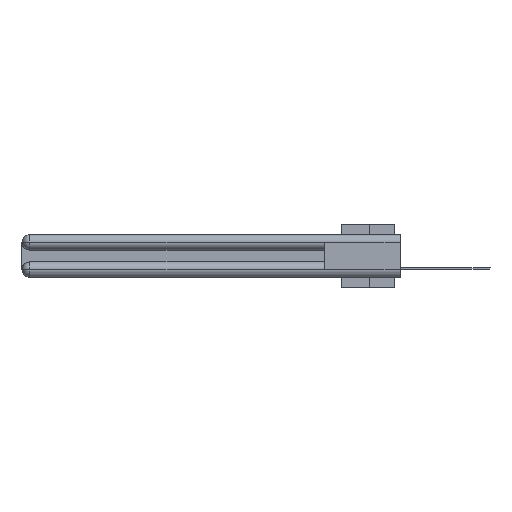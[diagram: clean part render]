
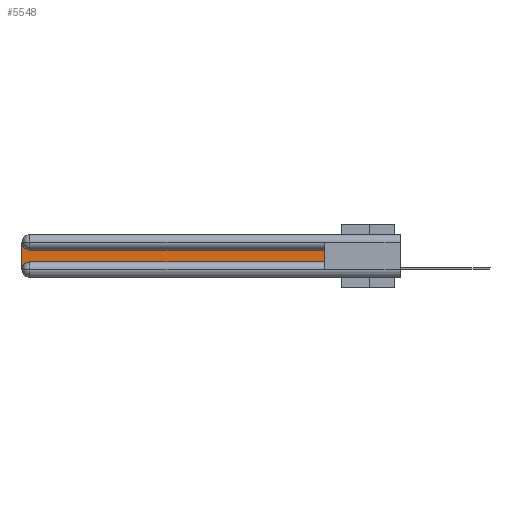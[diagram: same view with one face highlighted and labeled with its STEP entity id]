
A CAD part, left-side view. The second image highlights one B-rep face of the part: STEP entity #5548.
In plain terms, the highlighted planar face has unit normal (-1, 0, 0).
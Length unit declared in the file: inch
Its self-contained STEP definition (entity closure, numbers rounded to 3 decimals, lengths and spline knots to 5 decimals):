
#1590 = LINE ( 'NONE', #4368, #35063 ) ;
#1974 = CIRCLE ( 'NONE', #5161, 0.06 ) ;
#2086 = EDGE_LOOP ( 'NONE', ( #32346, #5162, #33347, #2254, #35032, #23874 ) ) ;
#2254 = ORIENTED_EDGE ( 'NONE', *, *, #33668, .T. ) ;
#3244 = DIRECTION ( 'NONE',  ( 0., -1., 0. ) ) ;
#3673 = EDGE_CURVE ( 'NONE', #18939, #28212, #23494, .T. ) ;
#4354 = VERTEX_POINT ( 'NONE', #37520 ) ;
#4368 = CARTESIAN_POINT ( 'NONE',  ( 0.075, 0.6, -0.2175 ) ) ;
#5161 = AXIS2_PLACEMENT_3D ( 'NONE', #16834, #28959, #37318 ) ;
#5162 = ORIENTED_EDGE ( 'NONE', *, *, #7898, .T. ) ;
#5548 = ADVANCED_FACE ( 'NONE', ( #9264 ), #30384, .F. ) ;
#6339 = VECTOR ( 'NONE', #36010, 39.37008 ) ;
#7898 = EDGE_CURVE ( 'NONE', #4354, #18939, #1974, .T. ) ;
#8536 = CARTESIAN_POINT ( 'NONE',  ( 0.075, 3., -0.2175 ) ) ;
#9244 = AXIS2_PLACEMENT_3D ( 'NONE', #24974, #36535, #33353 ) ;
#9264 = FACE_OUTER_BOUND ( 'NONE', #2086, .T. ) ;
#10869 = VERTEX_POINT ( 'NONE', #30142 ) ;
#11603 = LINE ( 'NONE', #23745, #30709 ) ;
#12467 = CARTESIAN_POINT ( 'NONE',  ( 0.075, 3., -0.1225 ) ) ;
#12664 = EDGE_CURVE ( 'NONE', #36570, #10869, #1590, .T. ) ;
#14847 = CARTESIAN_POINT ( 'NONE',  ( 0.075, 2.94, -0.2175 ) ) ;
#15653 = DIRECTION ( 'NONE',  ( 0., 0., -1. ) ) ;
#15775 = EDGE_CURVE ( 'NONE', #10869, #19020, #11603, .T. ) ;
#16488 = VECTOR ( 'NONE', #35612, 39.37008 ) ;
#16834 = CARTESIAN_POINT ( 'NONE',  ( 0.075, 2.94, -0.0625 ) ) ;
#16927 = LINE ( 'NONE', #17733, #6339 ) ;
#17733 = CARTESIAN_POINT ( 'NONE',  ( 0.075, 0.6, -0.1225 ) ) ;
#18939 = VERTEX_POINT ( 'NONE', #23603 ) ;
#19020 = VERTEX_POINT ( 'NONE', #32143 ) ;
#23277 = CIRCLE ( 'NONE', #9244, 0.06 ) ;
#23494 = LINE ( 'NONE', #8536, #16488 ) ;
#23603 = CARTESIAN_POINT ( 'NONE',  ( 0.075, 3., -0.0625 ) ) ;
#23745 = CARTESIAN_POINT ( 'NONE',  ( 0.075, 0.6, -0.2175 ) ) ;
#23874 = ORIENTED_EDGE ( 'NONE', *, *, #15775, .T. ) ;
#24974 = CARTESIAN_POINT ( 'NONE',  ( 0.075, 2.94, -0.2775 ) ) ;
#26121 = AXIS2_PLACEMENT_3D ( 'NONE', #12467, #33549, #15653 ) ;
#26284 = EDGE_CURVE ( 'NONE', #19020, #4354, #16927, .T. ) ;
#28212 = VERTEX_POINT ( 'NONE', #30406 ) ;
#28959 = DIRECTION ( 'NONE',  ( 1., 0., 0. ) ) ;
#30142 = CARTESIAN_POINT ( 'NONE',  ( 0.075, 0.6, -0.2175 ) ) ;
#30384 = PLANE ( 'NONE',  #26121 ) ;
#30406 = CARTESIAN_POINT ( 'NONE',  ( 0.075, 3., -0.2775 ) ) ;
#30709 = VECTOR ( 'NONE', #32889, 39.37008 ) ;
#32143 = CARTESIAN_POINT ( 'NONE',  ( 0.075, 0.6, -0.1225 ) ) ;
#32346 = ORIENTED_EDGE ( 'NONE', *, *, #26284, .T. ) ;
#32889 = DIRECTION ( 'NONE',  ( 0., 0., 1. ) ) ;
#33347 = ORIENTED_EDGE ( 'NONE', *, *, #3673, .T. ) ;
#33353 = DIRECTION ( 'NONE',  ( 0., 0., -1. ) ) ;
#33549 = DIRECTION ( 'NONE',  ( 1., 0., 0. ) ) ;
#33668 = EDGE_CURVE ( 'NONE', #28212, #36570, #23277, .T. ) ;
#35032 = ORIENTED_EDGE ( 'NONE', *, *, #12664, .T. ) ;
#35063 = VECTOR ( 'NONE', #3244, 39.37008 ) ;
#35612 = DIRECTION ( 'NONE',  ( 0., 0., -1. ) ) ;
#36010 = DIRECTION ( 'NONE',  ( 0., 1., 0. ) ) ;
#36535 = DIRECTION ( 'NONE',  ( 1., 0., 0. ) ) ;
#36570 = VERTEX_POINT ( 'NONE', #14847 ) ;
#37318 = DIRECTION ( 'NONE',  ( 0., 0., -1. ) ) ;
#37520 = CARTESIAN_POINT ( 'NONE',  ( 0.075, 2.94, -0.1225 ) ) ;
